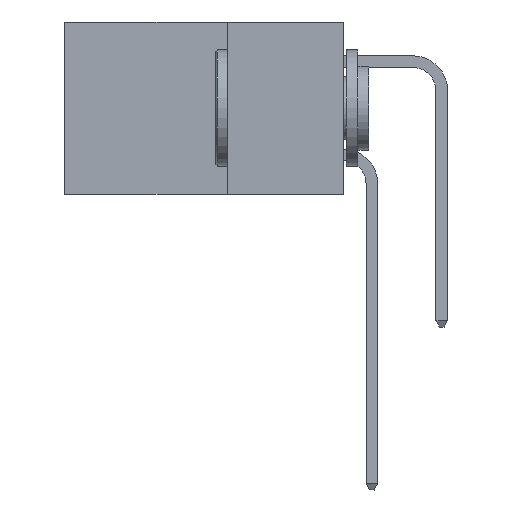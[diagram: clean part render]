
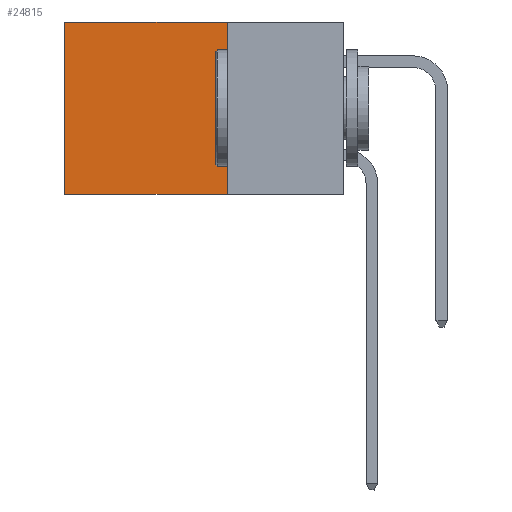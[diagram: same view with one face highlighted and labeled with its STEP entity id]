
A CAD part, left-side view. The second image highlights one B-rep face of the part: STEP entity #24815.
In plain terms, the highlighted planar face has unit normal (-1, 0, 0).
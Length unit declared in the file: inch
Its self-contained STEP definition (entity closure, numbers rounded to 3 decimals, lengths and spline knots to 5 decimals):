
#937 = PLANE ( 'NONE',  #19930 ) ;
#5140 = ORIENTED_EDGE ( 'NONE', *, *, #18500, .F. ) ;
#5798 = CARTESIAN_POINT ( 'NONE',  ( 0.298, 0.6, -0.37 ) ) ;
#8514 = VERTEX_POINT ( 'NONE', #13841 ) ;
#8712 = VERTEX_POINT ( 'NONE', #9779 ) ;
#9084 = DIRECTION ( 'NONE',  ( 0., 0., -1. ) ) ;
#9779 = CARTESIAN_POINT ( 'NONE',  ( 0.298, 0.25, 0. ) ) ;
#9836 = LINE ( 'NONE', #24600, #21686 ) ;
#10538 = DIRECTION ( 'NONE',  ( 1., 0., 0. ) ) ;
#11163 = ORIENTED_EDGE ( 'NONE', *, *, #29541, .T. ) ;
#12460 = DIRECTION ( 'NONE',  ( 0., 1., 0. ) ) ;
#13841 = CARTESIAN_POINT ( 'NONE',  ( 0.298, 0.25, -0.37 ) ) ;
#15037 = CARTESIAN_POINT ( 'NONE',  ( 0.298, 0.25, -0.37 ) ) ;
#15242 = DIRECTION ( 'NONE',  ( 0., 0., -1. ) ) ;
#18500 = EDGE_CURVE ( 'NONE', #8514, #21426, #23167, .T. ) ;
#18544 = EDGE_CURVE ( 'NONE', #8712, #8514, #9836, .T. ) ;
#19020 = VECTOR ( 'NONE', #9084, 39.37008 ) ;
#19800 = CARTESIAN_POINT ( 'NONE',  ( 0.298, 0.6, 0. ) ) ;
#19930 = AXIS2_PLACEMENT_3D ( 'NONE', #24643, #10538, #26972 ) ;
#20732 = EDGE_CURVE ( 'NONE', #8712, #20803, #29853, .T. ) ;
#20803 = VERTEX_POINT ( 'NONE', #19800 ) ;
#21426 = VERTEX_POINT ( 'NONE', #5798 ) ;
#21686 = VECTOR ( 'NONE', #15242, 39.37008 ) ;
#22176 = DIRECTION ( 'NONE',  ( 0., 1., 0. ) ) ;
#23033 = VECTOR ( 'NONE', #12460, 39.37008 ) ;
#23167 = LINE ( 'NONE', #15037, #23875 ) ;
#23301 = ORIENTED_EDGE ( 'NONE', *, *, #18544, .F. ) ;
#23343 = ORIENTED_EDGE ( 'NONE', *, *, #20732, .T. ) ;
#23875 = VECTOR ( 'NONE', #22176, 39.37008 ) ;
#24600 = CARTESIAN_POINT ( 'NONE',  ( 0.298, 0.25, 0. ) ) ;
#24643 = CARTESIAN_POINT ( 'NONE',  ( 0.298, 0.25, 0. ) ) ;
#24815 = ADVANCED_FACE ( 'NONE', ( #25816 ), #937, .F. ) ;
#25235 = LINE ( 'NONE', #27800, #19020 ) ;
#25816 = FACE_OUTER_BOUND ( 'NONE', #29417, .T. ) ;
#26972 = DIRECTION ( 'NONE',  ( 0., 0., -1. ) ) ;
#27800 = CARTESIAN_POINT ( 'NONE',  ( 0.298, 0.6, 0. ) ) ;
#28826 = CARTESIAN_POINT ( 'NONE',  ( 0.298, 0.25, 0. ) ) ;
#29417 = EDGE_LOOP ( 'NONE', ( #11163, #5140, #23301, #23343 ) ) ;
#29541 = EDGE_CURVE ( 'NONE', #20803, #21426, #25235, .T. ) ;
#29853 = LINE ( 'NONE', #28826, #23033 ) ;
